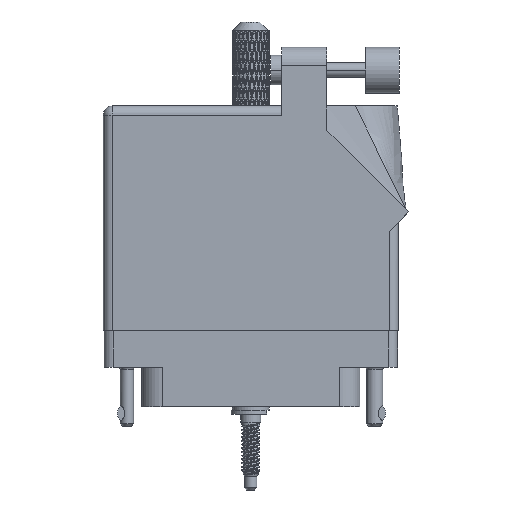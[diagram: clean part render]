
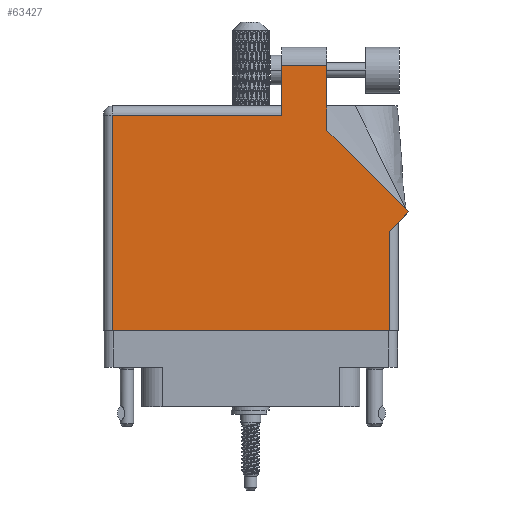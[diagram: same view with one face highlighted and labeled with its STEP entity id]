
A CAD part, front view. The second image highlights one B-rep face of the part: STEP entity #63427.
In plain terms, the highlighted face is planar.
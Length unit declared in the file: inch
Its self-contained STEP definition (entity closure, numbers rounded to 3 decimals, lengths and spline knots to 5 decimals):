
#165 = DIRECTION ( 'NONE',  ( 0., 1., 0. ) ) ;
#717 = VECTOR ( 'NONE', #74191, 39.37008 ) ;
#828 = ORIENTED_EDGE ( 'NONE', *, *, #67795, .T. ) ;
#1638 = LINE ( 'NONE', #35829, #75460 ) ;
#6206 = CARTESIAN_POINT ( 'NONE',  ( 0.212, 1.705, 0.455 ) ) ;
#6353 = ORIENTED_EDGE ( 'NONE', *, *, #104934, .T. ) ;
#7739 = CARTESIAN_POINT ( 'NONE',  ( -1.005, -0.1, 0.455 ) ) ;
#12247 = CARTESIAN_POINT ( 'NONE',  ( 0.212, 1.705, 0.455 ) ) ;
#12531 = VERTEX_POINT ( 'NONE', #30746 ) ;
#15458 = EDGE_CURVE ( 'NONE', #59329, #55109, #66285, .T. ) ;
#17280 = FACE_OUTER_BOUND ( 'NONE', #88516, .T. ) ;
#17534 = VECTOR ( 'NONE', #90898, 39.37008 ) ;
#18970 = VECTOR ( 'NONE', #63972, 39.37008 ) ;
#20229 = CARTESIAN_POINT ( 'NONE',  ( 1.005, 0.637, 0.455 ) ) ;
#20864 = AXIS2_PLACEMENT_3D ( 'NONE', #93422, #33109, #58222 ) ;
#21959 = EDGE_CURVE ( 'NONE', #35664, #84151, #86816, .T. ) ;
#22504 = CARTESIAN_POINT ( 'NONE',  ( -0.943, 1.368, 0.455 ) ) ;
#23458 = VECTOR ( 'NONE', #32648, 39.37008 ) ;
#26117 = CARTESIAN_POINT ( 'NONE',  ( 0.943, 0.575, 0.455 ) ) ;
#29932 = CARTESIAN_POINT ( 'NONE',  ( 0.212, 1.43, 0.455 ) ) ;
#30746 = CARTESIAN_POINT ( 'NONE',  ( 0.519, 1.705, 0.455 ) ) ;
#32648 = DIRECTION ( 'NONE',  ( 0., -1., 0. ) ) ;
#32914 = VECTOR ( 'NONE', #37641, 39.37008 ) ;
#33109 = DIRECTION ( 'NONE',  ( 0., 0., -1. ) ) ;
#35664 = VERTEX_POINT ( 'NONE', #107562 ) ;
#35829 = CARTESIAN_POINT ( 'NONE',  ( -1.005, 1.368, 0.455 ) ) ;
#37641 = DIRECTION ( 'NONE',  ( -0.707, 0.707, 0. ) ) ;
#39275 = ORIENTED_EDGE ( 'NONE', *, *, #77932, .T. ) ;
#40523 = LINE ( 'NONE', #20229, #95448 ) ;
#41898 = EDGE_CURVE ( 'NONE', #47483, #12531, #67857, .T. ) ;
#45571 = CARTESIAN_POINT ( 'NONE',  ( 1.07571, 0.70771, 0.455 ) ) ;
#46604 = CARTESIAN_POINT ( 'NONE',  ( 1.07571, 0.70771, 0.455 ) ) ;
#47483 = VERTEX_POINT ( 'NONE', #80554 ) ;
#52516 = LINE ( 'NONE', #29932, #18970 ) ;
#53124 = CARTESIAN_POINT ( 'NONE',  ( 0.212, 1.368, 0.455 ) ) ;
#54000 = ORIENTED_EDGE ( 'NONE', *, *, #21959, .T. ) ;
#55109 = VERTEX_POINT ( 'NONE', #100214 ) ;
#55902 = CARTESIAN_POINT ( 'NONE',  ( 0.519, 1.26442, 0.455 ) ) ;
#58222 = DIRECTION ( 'NONE',  ( -1., 0., 0. ) ) ;
#58705 = VECTOR ( 'NONE', #165, 39.37008 ) ;
#59329 = VERTEX_POINT ( 'NONE', #22504 ) ;
#63427 = ADVANCED_FACE ( 'NONE', ( #17280 ), #93038, .F. ) ;
#63972 = DIRECTION ( 'NONE',  ( 0., -1., 0. ) ) ;
#65262 = LINE ( 'NONE', #7739, #100111 ) ;
#66285 = LINE ( 'NONE', #92925, #23458 ) ;
#67795 = EDGE_CURVE ( 'NONE', #90458, #59329, #1638, .T. ) ;
#67857 = LINE ( 'NONE', #55902, #717 ) ;
#70571 = ORIENTED_EDGE ( 'NONE', *, *, #107254, .T. ) ;
#71223 = ORIENTED_EDGE ( 'NONE', *, *, #91249, .T. ) ;
#74191 = DIRECTION ( 'NONE',  ( 0., 1., 0. ) ) ;
#75460 = VECTOR ( 'NONE', #78775, 39.37008 ) ;
#77932 = EDGE_CURVE ( 'NONE', #99822, #47483, #86507, .T. ) ;
#78775 = DIRECTION ( 'NONE',  ( -1., 0., 0. ) ) ;
#80061 = DIRECTION ( 'NONE',  ( 0.707, 0.707, 0. ) ) ;
#80554 = CARTESIAN_POINT ( 'NONE',  ( 0.519, 1.26442, 0.455 ) ) ;
#83380 = ORIENTED_EDGE ( 'NONE', *, *, #15458, .T. ) ;
#84151 = VERTEX_POINT ( 'NONE', #26117 ) ;
#85266 = DIRECTION ( 'NONE',  ( 1., 0., 0. ) ) ;
#85755 = VERTEX_POINT ( 'NONE', #6206 ) ;
#86507 = LINE ( 'NONE', #46604, #32914 ) ;
#86718 = CARTESIAN_POINT ( 'NONE',  ( 0.943, 0.637, 0.455 ) ) ;
#86816 = LINE ( 'NONE', #86718, #58705 ) ;
#88516 = EDGE_LOOP ( 'NONE', ( #97244, #70571, #6353, #828, #83380, #103843, #54000, #71223, #39275 ) ) ;
#90458 = VERTEX_POINT ( 'NONE', #53124 ) ;
#90898 = DIRECTION ( 'NONE',  ( -1., 0., 0. ) ) ;
#91249 = EDGE_CURVE ( 'NONE', #84151, #99822, #40523, .T. ) ;
#92925 = CARTESIAN_POINT ( 'NONE',  ( -0.943, -0.1, 0.455 ) ) ;
#93038 = PLANE ( 'NONE',  #20864 ) ;
#93422 = CARTESIAN_POINT ( 'NONE',  ( -1.005, 1.43, 0.455 ) ) ;
#95448 = VECTOR ( 'NONE', #80061, 39.37008 ) ;
#96283 = EDGE_CURVE ( 'NONE', #55109, #35664, #65262, .T. ) ;
#97244 = ORIENTED_EDGE ( 'NONE', *, *, #41898, .T. ) ;
#99822 = VERTEX_POINT ( 'NONE', #45571 ) ;
#100111 = VECTOR ( 'NONE', #85266, 39.37008 ) ;
#100214 = CARTESIAN_POINT ( 'NONE',  ( -0.943, -0.1, 0.455 ) ) ;
#103843 = ORIENTED_EDGE ( 'NONE', *, *, #96283, .T. ) ;
#104934 = EDGE_CURVE ( 'NONE', #85755, #90458, #52516, .T. ) ;
#107254 = EDGE_CURVE ( 'NONE', #12531, #85755, #108614, .T. ) ;
#107562 = CARTESIAN_POINT ( 'NONE',  ( 0.943, -0.1, 0.455 ) ) ;
#108614 = LINE ( 'NONE', #12247, #17534 ) ;
